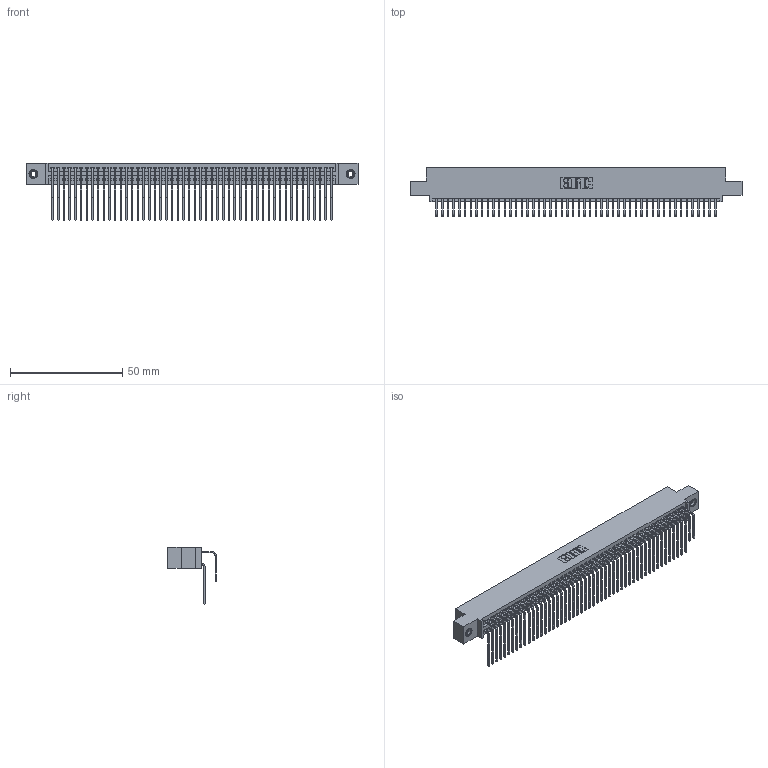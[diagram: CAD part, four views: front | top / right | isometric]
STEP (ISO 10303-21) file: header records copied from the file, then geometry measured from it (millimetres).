
FILE_DESCRIPTION (( 'STEP AP203' ), '1' );
FILE_NAME ('395-100-558-508.STEP', '2019-10-26T16:39:30', ( '' ), ( '' ), 'SwSTEP 2.0', 'SolidWorks 2016', '' );
FILE_SCHEMA (( 'CONFIG_CONTROL_DESIGN' ));
Length unit declared in the file: inch
Products named in the file (5): 395-100-558-508; 345 Part_0.110 Offset - 0.156 Dia-TI; 345-292-001_558 559 Tail - 1; 345-292-001_558 Tail - 2; 345-250-001_345-250-003-102
Assembly tree (103 placements, depth 2):
  395-100-558-508
    345 Part_0.110 Offset - 0.156 Dia-TI
    345-292-001_558 559 Tail - 1  x50
    345-292-001_558 Tail - 2  x50
    345-250-001_345-250-003-102  x2
Bounding box: 148.21 x 21.83 x 25.53 mm (x, y, z)
Volume: 14968.4 mm3; surface area: 25099.7 mm2
Topology: 103 solids, 103 shells, 5390 faces, 15989 edges, 10518 vertices
Faces by surface type: plane 3616, cylinder 1758, cone 12, torus 4
Entity records: 41124 total; most frequent: CARTESIAN_POINT 6914, ORIENTED_EDGE 6790, DIRECTION 6085, EDGE_CURVE 3395, LINE 3003, VECTOR 3003, VERTEX_POINT 2256, AXIS2_PLACEMENT_3D 1541
